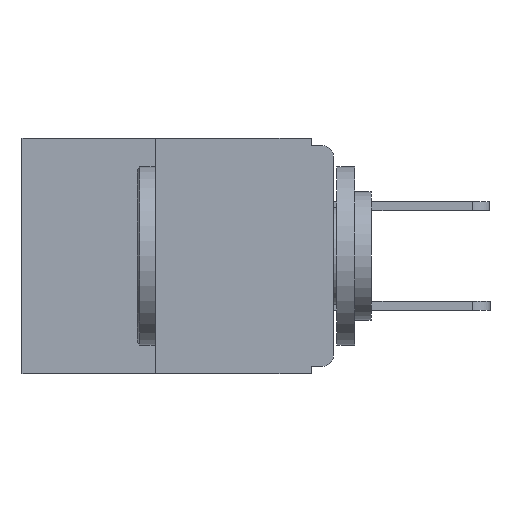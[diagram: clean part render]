
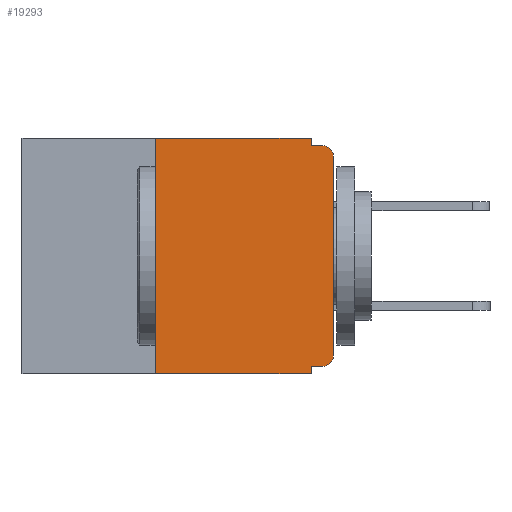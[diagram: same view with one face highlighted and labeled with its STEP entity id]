
A CAD part, left-side view. The second image highlights one B-rep face of the part: STEP entity #19293.
In plain terms, the highlighted planar face has unit normal (-1, 0, 0).
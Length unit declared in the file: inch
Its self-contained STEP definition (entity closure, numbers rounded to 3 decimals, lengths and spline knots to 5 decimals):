
#191 = VECTOR ( 'NONE', #19133, 39.37008 ) ;
#311 = DIRECTION ( 'NONE',  ( 0., 0., -1. ) ) ;
#529 = DIRECTION ( 'NONE',  ( 1., 0., 0. ) ) ;
#805 = CIRCLE ( 'NONE', #21840, 0.015 ) ;
#885 = EDGE_LOOP ( 'NONE', ( #1659, #3563, #21925, #23372, #22122, #3139, #17860, #7789, #10250, #16243 ) ) ;
#1330 = VECTOR ( 'NONE', #14628, 39.37008 ) ;
#1659 = ORIENTED_EDGE ( 'NONE', *, *, #22537, .T. ) ;
#2984 = CARTESIAN_POINT ( 'NONE',  ( 0., 0., -0.305 ) ) ;
#3139 = ORIENTED_EDGE ( 'NONE', *, *, #14168, .F. ) ;
#3494 = DIRECTION ( 'NONE',  ( 0., 1., 0. ) ) ;
#3563 = ORIENTED_EDGE ( 'NONE', *, *, #25978, .T. ) ;
#3805 = CARTESIAN_POINT ( 'NONE',  ( 0., 0., -0.01 ) ) ;
#3979 = CARTESIAN_POINT ( 'NONE',  ( 0., 0.031, -0.32 ) ) ;
#4038 = CARTESIAN_POINT ( 'NONE',  ( 0., 0.031, 0. ) ) ;
#4553 = DIRECTION ( 'NONE',  ( 0., 0., -1. ) ) ;
#5071 = DIRECTION ( 'NONE',  ( 0., 0., 1. ) ) ;
#6648 = VERTEX_POINT ( 'NONE', #21464 ) ;
#6664 = EDGE_CURVE ( 'NONE', #15000, #14361, #8719, .T. ) ;
#6797 = DIRECTION ( 'NONE',  ( -1., 0., 0. ) ) ;
#6885 = VECTOR ( 'NONE', #4553, 39.37008 ) ;
#7536 = VERTEX_POINT ( 'NONE', #8725 ) ;
#7580 = LINE ( 'NONE', #12353, #1330 ) ;
#7789 = ORIENTED_EDGE ( 'NONE', *, *, #8112, .F. ) ;
#8112 = EDGE_CURVE ( 'NONE', #20805, #27194, #24852, .T. ) ;
#8457 = CARTESIAN_POINT ( 'NONE',  ( 0., 0.25, 0. ) ) ;
#8719 = LINE ( 'NONE', #14706, #19364 ) ;
#8725 = CARTESIAN_POINT ( 'NONE',  ( 0., 0.015, -0.32 ) ) ;
#8811 = DIRECTION ( 'NONE',  ( 0., 0., -1. ) ) ;
#9618 = EDGE_CURVE ( 'NONE', #21547, #27194, #25791, .T. ) ;
#10250 = ORIENTED_EDGE ( 'NONE', *, *, #28880, .F. ) ;
#10281 = DIRECTION ( 'NONE',  ( 0., -1., 0. ) ) ;
#10419 = EDGE_CURVE ( 'NONE', #20649, #6648, #26413, .T. ) ;
#10782 = DIRECTION ( 'NONE',  ( 0., -1., 0. ) ) ;
#12280 = CARTESIAN_POINT ( 'NONE',  ( 0., 0.437, -0.33 ) ) ;
#12353 = CARTESIAN_POINT ( 'NONE',  ( 0., 0.25, -0.33 ) ) ;
#13129 = AXIS2_PLACEMENT_3D ( 'NONE', #14320, #529, #16595 ) ;
#14103 = DIRECTION ( 'NONE',  ( -1., 0., 0. ) ) ;
#14168 = EDGE_CURVE ( 'NONE', #21547, #15000, #7580, .T. ) ;
#14320 = CARTESIAN_POINT ( 'NONE',  ( 0., 0.437, 0. ) ) ;
#14361 = VERTEX_POINT ( 'NONE', #15123 ) ;
#14628 = DIRECTION ( 'NONE',  ( 0., 0., 1. ) ) ;
#14640 = FACE_OUTER_BOUND ( 'NONE', #885, .T. ) ;
#14703 = VECTOR ( 'NONE', #3494, 39.37008 ) ;
#14706 = CARTESIAN_POINT ( 'NONE',  ( 0., 0.437, 0. ) ) ;
#15000 = VERTEX_POINT ( 'NONE', #8457 ) ;
#15123 = CARTESIAN_POINT ( 'NONE',  ( 0., 0.031, 0. ) ) ;
#15681 = EDGE_CURVE ( 'NONE', #14361, #20649, #26427, .T. ) ;
#16243 = ORIENTED_EDGE ( 'NONE', *, *, #21611, .T. ) ;
#16595 = DIRECTION ( 'NONE',  ( 0., 0., -1. ) ) ;
#17860 = ORIENTED_EDGE ( 'NONE', *, *, #9618, .T. ) ;
#18211 = CARTESIAN_POINT ( 'NONE',  ( 0., 0.031, -0.33 ) ) ;
#18800 = PLANE ( 'NONE',  #13129 ) ;
#19133 = DIRECTION ( 'NONE',  ( 0., -1., 0. ) ) ;
#19293 = ADVANCED_FACE ( 'NONE', ( #14640 ), #18800, .F. ) ;
#19341 = VERTEX_POINT ( 'NONE', #2984 ) ;
#19364 = VECTOR ( 'NONE', #10281, 39.37008 ) ;
#20251 = CIRCLE ( 'NONE', #22296, 0.015 ) ;
#20416 = CARTESIAN_POINT ( 'NONE',  ( 0., 0.015, -0.305 ) ) ;
#20606 = VECTOR ( 'NONE', #10782, 39.37008 ) ;
#20619 = VECTOR ( 'NONE', #8811, 39.37008 ) ;
#20649 = VERTEX_POINT ( 'NONE', #23828 ) ;
#20758 = LINE ( 'NONE', #23829, #14703 ) ;
#20805 = VERTEX_POINT ( 'NONE', #3979 ) ;
#21045 = VERTEX_POINT ( 'NONE', #25143 ) ;
#21400 = CARTESIAN_POINT ( 'NONE',  ( 0., 0.031, -0.33 ) ) ;
#21464 = CARTESIAN_POINT ( 'NONE',  ( 0., 0.015, -0.01 ) ) ;
#21547 = VERTEX_POINT ( 'NONE', #28820 ) ;
#21611 = EDGE_CURVE ( 'NONE', #7536, #19341, #20251, .T. ) ;
#21840 = AXIS2_PLACEMENT_3D ( 'NONE', #27456, #14103, #311 ) ;
#21925 = ORIENTED_EDGE ( 'NONE', *, *, #10419, .F. ) ;
#22122 = ORIENTED_EDGE ( 'NONE', *, *, #6664, .F. ) ;
#22296 = AXIS2_PLACEMENT_3D ( 'NONE', #20416, #6797, #22661 ) ;
#22537 = EDGE_CURVE ( 'NONE', #19341, #21045, #23311, .T. ) ;
#22661 = DIRECTION ( 'NONE',  ( 0., 0., -1. ) ) ;
#23215 = CARTESIAN_POINT ( 'NONE',  ( 0., 0., 0. ) ) ;
#23311 = LINE ( 'NONE', #23215, #28405 ) ;
#23372 = ORIENTED_EDGE ( 'NONE', *, *, #15681, .F. ) ;
#23828 = CARTESIAN_POINT ( 'NONE',  ( 0., 0.031, -0.01 ) ) ;
#23829 = CARTESIAN_POINT ( 'NONE',  ( 0., 0., -0.32 ) ) ;
#24852 = LINE ( 'NONE', #18211, #6885 ) ;
#25143 = CARTESIAN_POINT ( 'NONE',  ( 0., 0., -0.025 ) ) ;
#25791 = LINE ( 'NONE', #12280, #191 ) ;
#25978 = EDGE_CURVE ( 'NONE', #21045, #6648, #805, .T. ) ;
#26413 = LINE ( 'NONE', #3805, #20606 ) ;
#26427 = LINE ( 'NONE', #4038, #20619 ) ;
#27194 = VERTEX_POINT ( 'NONE', #21400 ) ;
#27456 = CARTESIAN_POINT ( 'NONE',  ( 0., 0.015, -0.025 ) ) ;
#28405 = VECTOR ( 'NONE', #5071, 39.37008 ) ;
#28820 = CARTESIAN_POINT ( 'NONE',  ( 0., 0.25, -0.33 ) ) ;
#28880 = EDGE_CURVE ( 'NONE', #7536, #20805, #20758, .T. ) ;
